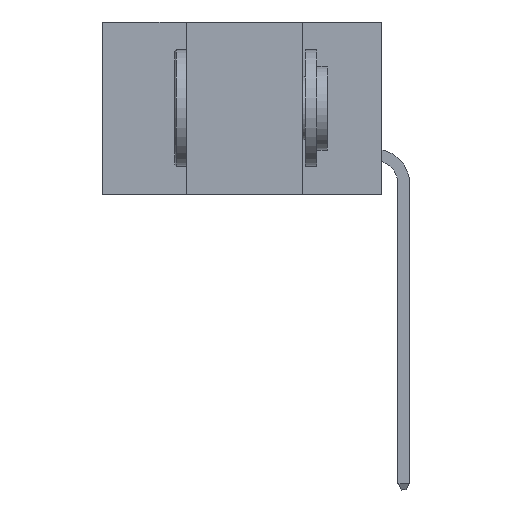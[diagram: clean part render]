
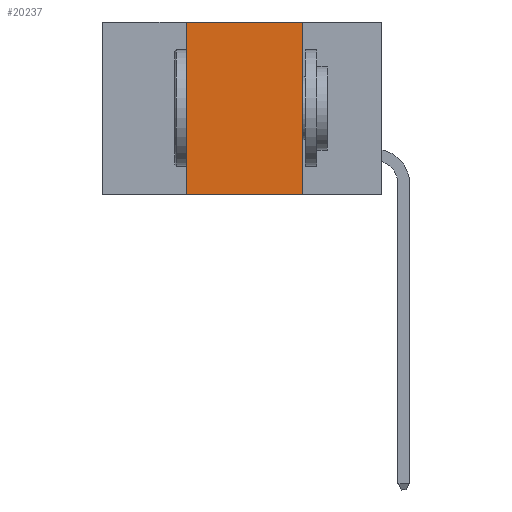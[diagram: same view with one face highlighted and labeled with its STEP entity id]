
A CAD part, left-side view. The second image highlights one B-rep face of the part: STEP entity #20237.
In plain terms, the highlighted planar face has unit normal (-1, 0, 0).
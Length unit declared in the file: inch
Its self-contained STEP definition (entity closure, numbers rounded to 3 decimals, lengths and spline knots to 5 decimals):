
#5755 = LINE ( 'NONE', #34131, #19663 ) ;
#5833 = VERTEX_POINT ( 'NONE', #9939 ) ;
#7196 = FACE_OUTER_BOUND ( 'NONE', #25953, .T. ) ;
#8050 = CARTESIAN_POINT ( 'NONE',  ( 0., 0.6, 0. ) ) ;
#9659 = VECTOR ( 'NONE', #30025, 39.37008 ) ;
#9939 = CARTESIAN_POINT ( 'NONE',  ( 0., 0.42, 0. ) ) ;
#10864 = DIRECTION ( 'NONE',  ( 0., 0., -1. ) ) ;
#11398 = LINE ( 'NONE', #13490, #9659 ) ;
#13056 = ORIENTED_EDGE ( 'NONE', *, *, #21806, .F. ) ;
#13490 = CARTESIAN_POINT ( 'NONE',  ( 0., 0.17, 0. ) ) ;
#14034 = LINE ( 'NONE', #18110, #19676 ) ;
#14417 = EDGE_CURVE ( 'NONE', #18228, #20057, #11398, .T. ) ;
#14880 = DIRECTION ( 'NONE',  ( 0., -1., 0. ) ) ;
#15341 = AXIS2_PLACEMENT_3D ( 'NONE', #8050, #27475, #10864 ) ;
#17612 = CARTESIAN_POINT ( 'NONE',  ( 0., 0.17, 0. ) ) ;
#18110 = CARTESIAN_POINT ( 'NONE',  ( 0., 0.42, 0. ) ) ;
#18228 = VERTEX_POINT ( 'NONE', #17612 ) ;
#19663 = VECTOR ( 'NONE', #14880, 39.37008 ) ;
#19668 = CARTESIAN_POINT ( 'NONE',  ( 0., 0.42, -0.37 ) ) ;
#19676 = VECTOR ( 'NONE', #20907, 39.37008 ) ;
#20057 = VERTEX_POINT ( 'NONE', #21062 ) ;
#20237 = ADVANCED_FACE ( 'NONE', ( #7196 ), #35477, .F. ) ;
#20907 = DIRECTION ( 'NONE',  ( 0., 0., 1. ) ) ;
#21062 = CARTESIAN_POINT ( 'NONE',  ( 0., 0.17, -0.37 ) ) ;
#21806 = EDGE_CURVE ( 'NONE', #5833, #18228, #5755, .T. ) ;
#25953 = EDGE_LOOP ( 'NONE', ( #29068, #13056, #35390, #30365 ) ) ;
#27475 = DIRECTION ( 'NONE',  ( 1., 0., 0. ) ) ;
#29068 = ORIENTED_EDGE ( 'NONE', *, *, #14417, .F. ) ;
#30025 = DIRECTION ( 'NONE',  ( 0., 0., -1. ) ) ;
#30365 = ORIENTED_EDGE ( 'NONE', *, *, #32087, .T. ) ;
#31240 = VECTOR ( 'NONE', #34705, 39.37008 ) ;
#31414 = EDGE_CURVE ( 'NONE', #35563, #5833, #14034, .T. ) ;
#31981 = CARTESIAN_POINT ( 'NONE',  ( 0., 0.6, -0.37 ) ) ;
#32070 = LINE ( 'NONE', #31981, #31240 ) ;
#32087 = EDGE_CURVE ( 'NONE', #35563, #20057, #32070, .T. ) ;
#34131 = CARTESIAN_POINT ( 'NONE',  ( 0., 0.6, 0. ) ) ;
#34705 = DIRECTION ( 'NONE',  ( 0., -1., 0. ) ) ;
#35390 = ORIENTED_EDGE ( 'NONE', *, *, #31414, .F. ) ;
#35477 = PLANE ( 'NONE',  #15341 ) ;
#35563 = VERTEX_POINT ( 'NONE', #19668 ) ;
